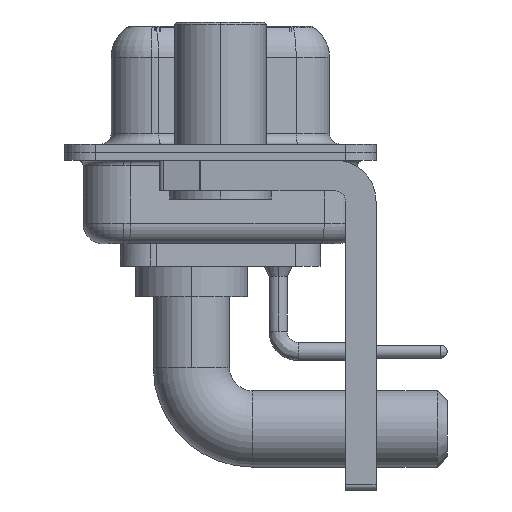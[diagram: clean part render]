
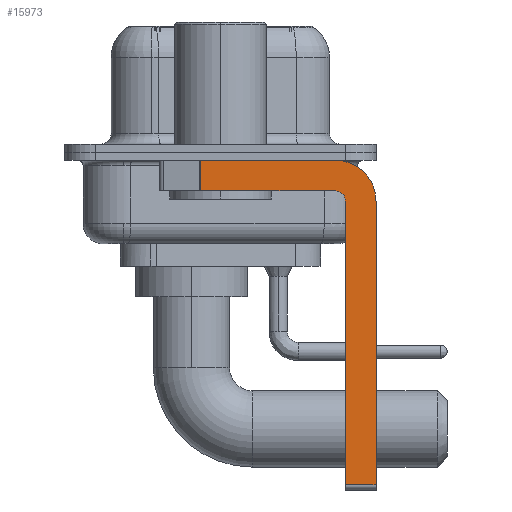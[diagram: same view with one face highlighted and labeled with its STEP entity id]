
A CAD part, left-side view. The second image highlights one B-rep face of the part: STEP entity #15973.
In plain terms, the highlighted planar face has unit normal (-1, 0, 0).
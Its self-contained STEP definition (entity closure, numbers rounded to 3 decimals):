
#296 = EDGE_CURVE ( 'NONE', #18886, #1061, #5895, .T. ) ;
#600 = DIRECTION ( 'NONE',  ( 0., 0., -1. ) ) ;
#657 = DIRECTION ( 'NONE',  ( 0., 0., 1. ) ) ;
#923 = CARTESIAN_POINT ( 'NONE',  ( -2.9, 3., -0.4 ) ) ;
#1061 = VERTEX_POINT ( 'NONE', #21356 ) ;
#1210 = DIRECTION ( 'NONE',  ( 0., 0., -1. ) ) ;
#1305 = VERTEX_POINT ( 'NONE', #9736 ) ;
#1374 = CARTESIAN_POINT ( 'NONE',  ( -2.9, -7.65, -16.35 ) ) ;
#1384 = DIRECTION ( 'NONE',  ( 1., 0., 0. ) ) ;
#1445 = LINE ( 'NONE', #13941, #22114 ) ;
#1452 = ORIENTED_EDGE ( 'NONE', *, *, #18499, .F. ) ;
#2136 = LINE ( 'NONE', #7796, #20079 ) ;
#2932 = DIRECTION ( 'NONE',  ( 0., -1., 0. ) ) ;
#3165 = CIRCLE ( 'NONE', #11584, 2. ) ;
#4480 = ORIENTED_EDGE ( 'NONE', *, *, #18280, .F. ) ;
#4689 = ORIENTED_EDGE ( 'NONE', *, *, #296, .F. ) ;
#4748 = CARTESIAN_POINT ( 'NONE',  ( -2.9, -5.65, -2.4 ) ) ;
#5693 = FACE_OUTER_BOUND ( 'NONE', #23473, .T. ) ;
#5858 = VERTEX_POINT ( 'NONE', #9867 ) ;
#5895 = CIRCLE ( 'NONE', #17376, 0.5 ) ;
#6020 = LINE ( 'NONE', #13311, #12149 ) ;
#6892 = LINE ( 'NONE', #19716, #19459 ) ;
#6919 = PLANE ( 'NONE',  #14294 ) ;
#7181 = ORIENTED_EDGE ( 'NONE', *, *, #22563, .T. ) ;
#7796 = CARTESIAN_POINT ( 'NONE',  ( -2.9, -5.65, -1.9 ) ) ;
#7831 = DIRECTION ( 'NONE',  ( 0., 0., -1. ) ) ;
#8049 = CARTESIAN_POINT ( 'NONE',  ( -2.9, -5.65, -2.4 ) ) ;
#8143 = ORIENTED_EDGE ( 'NONE', *, *, #21757, .T. ) ;
#8636 = VERTEX_POINT ( 'NONE', #21728 ) ;
#9465 = DIRECTION ( 'NONE',  ( 0., 1., 0. ) ) ;
#9528 = CARTESIAN_POINT ( 'NONE',  ( -2.9, -6.15, -2.4 ) ) ;
#9736 = CARTESIAN_POINT ( 'NONE',  ( -2.9, -5.65, -0.4 ) ) ;
#9867 = CARTESIAN_POINT ( 'NONE',  ( -2.9, 0.978, -0.4 ) ) ;
#10509 = VECTOR ( 'NONE', #21076, 1000. ) ;
#10780 = ORIENTED_EDGE ( 'NONE', *, *, #13938, .F. ) ;
#11584 = AXIS2_PLACEMENT_3D ( 'NONE', #8049, #18723, #600 ) ;
#12146 = DIRECTION ( 'NONE',  ( -1., 0., 0. ) ) ;
#12149 = VECTOR ( 'NONE', #19307, 1000. ) ;
#13263 = VERTEX_POINT ( 'NONE', #1374 ) ;
#13311 = CARTESIAN_POINT ( 'NONE',  ( -2.9, -6.15, -16.6 ) ) ;
#13938 = EDGE_CURVE ( 'NONE', #17613, #13263, #20771, .T. ) ;
#13941 = CARTESIAN_POINT ( 'NONE',  ( -2.9, 0.978, -1.9 ) ) ;
#14294 = AXIS2_PLACEMENT_3D ( 'NONE', #18090, #1384, #16286 ) ;
#15251 = EDGE_CURVE ( 'NONE', #1305, #17613, #3165, .T. ) ;
#15817 = ORIENTED_EDGE ( 'NONE', *, *, #22084, .F. ) ;
#15973 = ADVANCED_FACE ( 'NONE', ( #5693 ), #6919, .F. ) ;
#16286 = DIRECTION ( 'NONE',  ( 0., 0., -1. ) ) ;
#17250 = VERTEX_POINT ( 'NONE', #22999 ) ;
#17376 = AXIS2_PLACEMENT_3D ( 'NONE', #4748, #12146, #657 ) ;
#17613 = VERTEX_POINT ( 'NONE', #21276 ) ;
#18090 = CARTESIAN_POINT ( 'NONE',  ( -2.9, -5.65, -2.4 ) ) ;
#18280 = EDGE_CURVE ( 'NONE', #1061, #8636, #2136, .T. ) ;
#18499 = EDGE_CURVE ( 'NONE', #5858, #1305, #22884, .T. ) ;
#18723 = DIRECTION ( 'NONE',  ( 1., 0., 0. ) ) ;
#18886 = VERTEX_POINT ( 'NONE', #9528 ) ;
#19307 = DIRECTION ( 'NONE',  ( 0., 0., 1. ) ) ;
#19459 = VECTOR ( 'NONE', #2932, 1000. ) ;
#19716 = CARTESIAN_POINT ( 'NONE',  ( -2.9, -5.65, -16.35 ) ) ;
#20079 = VECTOR ( 'NONE', #9465, 1000. ) ;
#20771 = LINE ( 'NONE', #22321, #22649 ) ;
#21076 = DIRECTION ( 'NONE',  ( 0., -1., 0. ) ) ;
#21276 = CARTESIAN_POINT ( 'NONE',  ( -2.9, -7.65, -2.4 ) ) ;
#21356 = CARTESIAN_POINT ( 'NONE',  ( -2.9, -5.65, -1.9 ) ) ;
#21639 = ORIENTED_EDGE ( 'NONE', *, *, #15251, .F. ) ;
#21728 = CARTESIAN_POINT ( 'NONE',  ( -2.9, 0.978, -1.9 ) ) ;
#21757 = EDGE_CURVE ( 'NONE', #5858, #8636, #1445, .T. ) ;
#22084 = EDGE_CURVE ( 'NONE', #17250, #18886, #6020, .T. ) ;
#22114 = VECTOR ( 'NONE', #1210, 1000. ) ;
#22321 = CARTESIAN_POINT ( 'NONE',  ( -2.9, -7.65, -2.4 ) ) ;
#22563 = EDGE_CURVE ( 'NONE', #17250, #13263, #6892, .T. ) ;
#22649 = VECTOR ( 'NONE', #7831, 1000. ) ;
#22884 = LINE ( 'NONE', #923, #10509 ) ;
#22999 = CARTESIAN_POINT ( 'NONE',  ( -2.9, -6.15, -16.35 ) ) ;
#23473 = EDGE_LOOP ( 'NONE', ( #1452, #8143, #4480, #4689, #15817, #7181, #10780, #21639 ) ) ;
